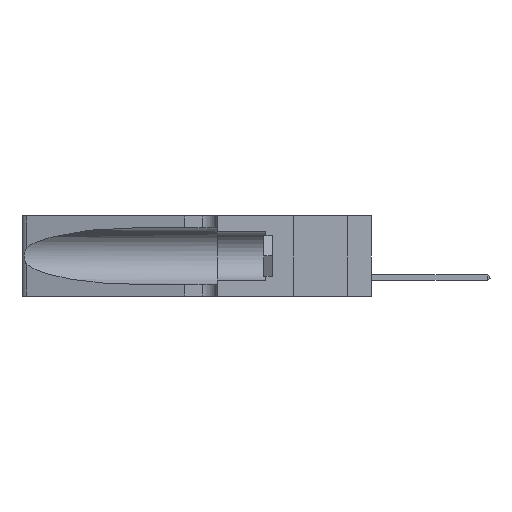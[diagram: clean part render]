
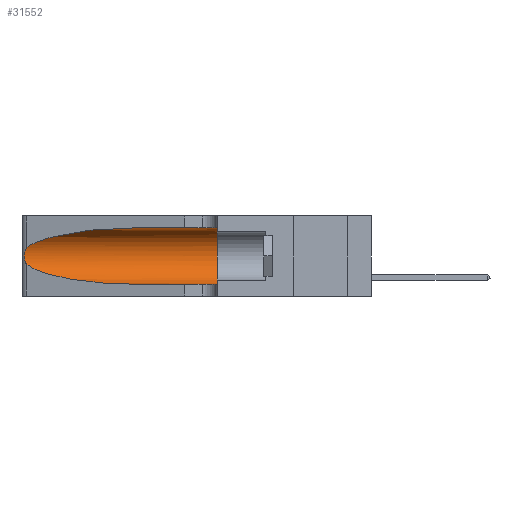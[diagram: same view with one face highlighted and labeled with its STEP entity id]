
A CAD part, left-side view. The second image highlights one B-rep face of the part: STEP entity #31552.
In plain terms, the highlighted cylindrical face has radius 3.308 mm (diameter 6.617 mm), a partial arc.
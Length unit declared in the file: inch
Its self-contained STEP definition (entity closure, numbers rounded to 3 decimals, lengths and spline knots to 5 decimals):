
#1838 = VERTEX_POINT ( 'NONE', #8980 ) ;
#2701 = CARTESIAN_POINT ( 'NONE',  ( 0.2373, 1.15595, 0.28018 ) ) ;
#5912 = CARTESIAN_POINT ( 'NONE',  ( 0.25856, 1.23593, 0.16098 ) ) ;
#6523 = CARTESIAN_POINT ( 'NONE',  ( 0.2373, 1.15595, 0.08982 ) ) ;
#6782 = ORIENTED_EDGE ( 'NONE', *, *, #15964, .T. ) ;
#8220 = CARTESIAN_POINT ( 'NONE',  ( 0.1305, 1.61858, 0.31525 ) ) ;
#8629 = CARTESIAN_POINT ( 'NONE',  ( 0.25487, 1.22718, 0.22369 ) ) ;
#8980 = CARTESIAN_POINT ( 'NONE',  ( 0.1305, 0.35, 0.05475 ) ) ;
#9409 = CARTESIAN_POINT ( 'NONE',  ( 0.26017, 1.23833, 0.17102 ) ) ;
#9475 = CARTESIAN_POINT ( 'NONE',  ( 0.1305, 0.72297, 0.05475 ) ) ;
#9765 = CARTESIAN_POINT ( 'NONE',  ( 0.25487, 1.22718, 0.22369 ) ) ;
#11094 =( BOUNDED_CURVE ( )  B_SPLINE_CURVE ( 3, ( #22842, #6523, #46445, #18628 ),
 .UNSPECIFIED., .F., .T. ) 
 B_SPLINE_CURVE_WITH_KNOTS ( ( 4, 4 ),
 ( 3.44316, 4.71239 ),
 .UNSPECIFIED. ) 
 CURVE ( )  GEOMETRIC_REPRESENTATION_ITEM ( )  RATIONAL_B_SPLINE_CURVE ( ( 1., 0.87, 0.87, 1. ) ) 
 REPRESENTATION_ITEM ( '' )  );
#11413 = B_SPLINE_CURVE_WITH_KNOTS ( 'NONE', 3,
 ( #9765, #29950, #13442, #41463, #37610, #37793, #17661, #21336, #9409, #5912, #49856, #25545, #41280, #45462 ),
 .UNSPECIFIED., .F., .F.,
 ( 4, 2, 2, 2, 2, 2, 4 ),
 ( 0., 0.00027, 0.00053, 0.00107, 0.0016, 0.00187, 0.00214 ),
 .UNSPECIFIED. ) ;
#11475 = VERTEX_POINT ( 'NONE', #16620 ) ;
#11596 = DIRECTION ( 'NONE',  ( 0., -1., 0. ) ) ;
#11809 =( BOUNDED_CURVE ( )  B_SPLINE_CURVE ( 3, ( #38614, #41888, #2701, #42480 ),
 .UNSPECIFIED., .F., .F. ) 
 B_SPLINE_CURVE_WITH_KNOTS ( ( 4, 4 ),
 ( 1.5708, 2.84003 ),
 .UNSPECIFIED. ) 
 CURVE ( )  GEOMETRIC_REPRESENTATION_ITEM ( )  RATIONAL_B_SPLINE_CURVE ( ( 1., 0.87, 0.87, 1. ) ) 
 REPRESENTATION_ITEM ( '' )  );
#12678 = CYLINDRICAL_SURFACE ( 'NONE', #31591, 0.13025 ) ;
#13442 = CARTESIAN_POINT ( 'NONE',  ( 0.25639, 1.23184, 0.21858 ) ) ;
#15964 = EDGE_CURVE ( 'NONE', #50170, #44418, #11809, .T. ) ;
#16620 = CARTESIAN_POINT ( 'NONE',  ( 0.1305, 0.35, 0.31525 ) ) ;
#17273 = CARTESIAN_POINT ( 'NONE',  ( 0.1305, 1.61858, 0.185 ) ) ;
#17661 = CARTESIAN_POINT ( 'NONE',  ( 0.26075, 1.23896, 0.19203 ) ) ;
#18628 = CARTESIAN_POINT ( 'NONE',  ( 0.1305, 0.72297, 0.05475 ) ) ;
#18803 = ORIENTED_EDGE ( 'NONE', *, *, #44751, .T. ) ;
#19593 = EDGE_CURVE ( 'NONE', #11475, #1838, #28647, .T. ) ;
#20201 = VECTOR ( 'NONE', #11596, 39.37008 ) ;
#21336 = CARTESIAN_POINT ( 'NONE',  ( 0.26075, 1.23896, 0.178 ) ) ;
#22842 = CARTESIAN_POINT ( 'NONE',  ( 0.25487, 1.22718, 0.14631 ) ) ;
#23114 = ORIENTED_EDGE ( 'NONE', *, *, #39803, .T. ) ;
#25199 = VERTEX_POINT ( 'NONE', #9475 ) ;
#25545 = CARTESIAN_POINT ( 'NONE',  ( 0.25639, 1.23186, 0.15144 ) ) ;
#25578 = CARTESIAN_POINT ( 'NONE',  ( 0.1305, 0.35, 0.185 ) ) ;
#26528 = DIRECTION ( 'NONE',  ( 0., 0., 1. ) ) ;
#27089 = ORIENTED_EDGE ( 'NONE', *, *, #19593, .F. ) ;
#27811 = FACE_OUTER_BOUND ( 'NONE', #50562, .T. ) ;
#27887 = CARTESIAN_POINT ( 'NONE',  ( 0.1305, 1.61858, 0.05475 ) ) ;
#28647 = CIRCLE ( 'NONE', #36188, 0.13025 ) ;
#29518 = EDGE_CURVE ( 'NONE', #50170, #11475, #49813, .T. ) ;
#29950 = CARTESIAN_POINT ( 'NONE',  ( 0.25555, 1.22994, 0.2215 ) ) ;
#30416 = ORIENTED_EDGE ( 'NONE', *, *, #29518, .F. ) ;
#31552 = ADVANCED_FACE ( 'NONE', ( #27811 ), #12678, .F. ) ;
#31591 = AXIS2_PLACEMENT_3D ( 'NONE', #17273, #40084, #44555 ) ;
#35880 = LINE ( 'NONE', #27887, #20201 ) ;
#36188 = AXIS2_PLACEMENT_3D ( 'NONE', #25578, #38953, #26528 ) ;
#37610 = CARTESIAN_POINT ( 'NONE',  ( 0.25854, 1.2359, 0.20912 ) ) ;
#37793 = CARTESIAN_POINT ( 'NONE',  ( 0.26018, 1.23835, 0.19895 ) ) ;
#38599 = ORIENTED_EDGE ( 'NONE', *, *, #47212, .T. ) ;
#38614 = CARTESIAN_POINT ( 'NONE',  ( 0.1305, 0.72297, 0.31525 ) ) ;
#38953 = DIRECTION ( 'NONE',  ( 0., 1., 0. ) ) ;
#39803 = EDGE_CURVE ( 'NONE', #44418, #41170, #11413, .T. ) ;
#40084 = DIRECTION ( 'NONE',  ( 0., -1., 0. ) ) ;
#41170 = VERTEX_POINT ( 'NONE', #47477 ) ;
#41280 = CARTESIAN_POINT ( 'NONE',  ( 0.25555, 1.22993, 0.14849 ) ) ;
#41463 = CARTESIAN_POINT ( 'NONE',  ( 0.25787, 1.23484, 0.2124 ) ) ;
#41888 = CARTESIAN_POINT ( 'NONE',  ( 0.18966, 0.96281, 0.31525 ) ) ;
#42480 = CARTESIAN_POINT ( 'NONE',  ( 0.25487, 1.22718, 0.22369 ) ) ;
#43567 = DIRECTION ( 'NONE',  ( 0., -1., 0. ) ) ;
#44418 = VERTEX_POINT ( 'NONE', #8629 ) ;
#44555 = DIRECTION ( 'NONE',  ( 0., 0., -1. ) ) ;
#44751 = EDGE_CURVE ( 'NONE', #41170, #25199, #11094, .T. ) ;
#45462 = CARTESIAN_POINT ( 'NONE',  ( 0.25487, 1.22718, 0.14631 ) ) ;
#46445 = CARTESIAN_POINT ( 'NONE',  ( 0.18966, 0.96281, 0.05475 ) ) ;
#47212 = EDGE_CURVE ( 'NONE', #25199, #1838, #35880, .T. ) ;
#47477 = CARTESIAN_POINT ( 'NONE',  ( 0.25487, 1.22718, 0.14631 ) ) ;
#48587 = VECTOR ( 'NONE', #43567, 39.37008 ) ;
#49813 = LINE ( 'NONE', #8220, #48587 ) ;
#49856 = CARTESIAN_POINT ( 'NONE',  ( 0.25789, 1.23486, 0.15765 ) ) ;
#49877 = CARTESIAN_POINT ( 'NONE',  ( 0.1305, 0.72297, 0.31525 ) ) ;
#50170 = VERTEX_POINT ( 'NONE', #49877 ) ;
#50562 = EDGE_LOOP ( 'NONE', ( #6782, #23114, #18803, #38599, #27089, #30416 ) ) ;
